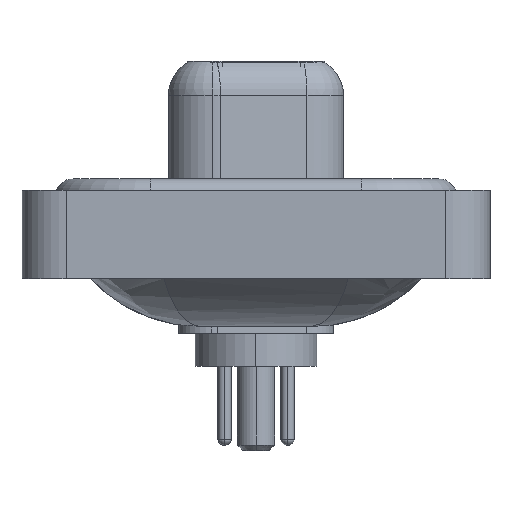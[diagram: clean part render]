
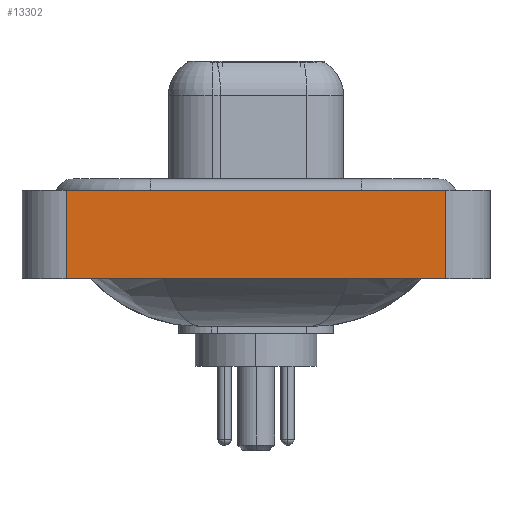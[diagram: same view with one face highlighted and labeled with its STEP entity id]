
A CAD part, left-side view. The second image highlights one B-rep face of the part: STEP entity #13302.
In plain terms, the highlighted planar face has unit normal (-1, 0, 0).
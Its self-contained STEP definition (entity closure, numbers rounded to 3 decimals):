
#218 = DIRECTION ( 'NONE',  ( 0., 0., 1. ) ) ;
#325 = CARTESIAN_POINT ( 'NONE',  ( -7.35, -8.55, -3.6 ) ) ;
#1033 = LINE ( 'NONE', #16639, #7321 ) ;
#1760 = VERTEX_POINT ( 'NONE', #18121 ) ;
#3500 = AXIS2_PLACEMENT_3D ( 'NONE', #325, #10678, #218 ) ;
#4315 = VERTEX_POINT ( 'NONE', #18154 ) ;
#4633 = DIRECTION ( 'NONE',  ( 0., -1., 0. ) ) ;
#6119 = CARTESIAN_POINT ( 'NONE',  ( -7.35, -8.55, -3.6 ) ) ;
#6165 = EDGE_CURVE ( 'NONE', #4315, #7845, #17936, .T. ) ;
#7161 = FACE_OUTER_BOUND ( 'NONE', #10248, .T. ) ;
#7321 = VECTOR ( 'NONE', #21753, 1000. ) ;
#7600 = EDGE_CURVE ( 'NONE', #21707, #7845, #7824, .T. ) ;
#7666 = EDGE_CURVE ( 'NONE', #1760, #21707, #8376, .T. ) ;
#7824 = LINE ( 'NONE', #6119, #19955 ) ;
#7845 = VERTEX_POINT ( 'NONE', #14286 ) ;
#8376 = LINE ( 'NONE', #20200, #11244 ) ;
#9298 = EDGE_CURVE ( 'NONE', #1760, #4315, #1033, .T. ) ;
#9301 = CARTESIAN_POINT ( 'NONE',  ( -7.35, -8.55, 0.4 ) ) ;
#9367 = VECTOR ( 'NONE', #16246, 1000. ) ;
#10027 = ORIENTED_EDGE ( 'NONE', *, *, #7600, .T. ) ;
#10248 = EDGE_LOOP ( 'NONE', ( #10027, #18637, #10885, #16505 ) ) ;
#10678 = DIRECTION ( 'NONE',  ( -1., 0., 0. ) ) ;
#10885 = ORIENTED_EDGE ( 'NONE', *, *, #9298, .F. ) ;
#11100 = CARTESIAN_POINT ( 'NONE',  ( -7.35, -8.55, -3.6 ) ) ;
#11244 = VECTOR ( 'NONE', #4633, 1000. ) ;
#13041 = DIRECTION ( 'NONE',  ( 0., 0., 1. ) ) ;
#13302 = ADVANCED_FACE ( 'NONE', ( #7161 ), #18975, .T. ) ;
#14286 = CARTESIAN_POINT ( 'NONE',  ( -7.35, -8.55, 0.4 ) ) ;
#16246 = DIRECTION ( 'NONE',  ( 0., -1., 0. ) ) ;
#16505 = ORIENTED_EDGE ( 'NONE', *, *, #7666, .T. ) ;
#16639 = CARTESIAN_POINT ( 'NONE',  ( -7.35, 8.55, -3.6 ) ) ;
#17936 = LINE ( 'NONE', #9301, #9367 ) ;
#18121 = CARTESIAN_POINT ( 'NONE',  ( -7.35, 8.55, -3.6 ) ) ;
#18154 = CARTESIAN_POINT ( 'NONE',  ( -7.35, 8.55, 0.4 ) ) ;
#18637 = ORIENTED_EDGE ( 'NONE', *, *, #6165, .F. ) ;
#18975 = PLANE ( 'NONE',  #3500 ) ;
#19955 = VECTOR ( 'NONE', #13041, 1000. ) ;
#20200 = CARTESIAN_POINT ( 'NONE',  ( -7.35, -8.55, -3.6 ) ) ;
#21707 = VERTEX_POINT ( 'NONE', #11100 ) ;
#21753 = DIRECTION ( 'NONE',  ( 0., 0., 1. ) ) ;
